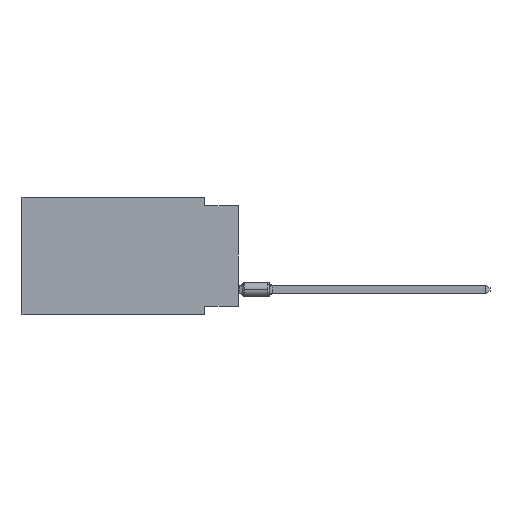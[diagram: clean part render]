
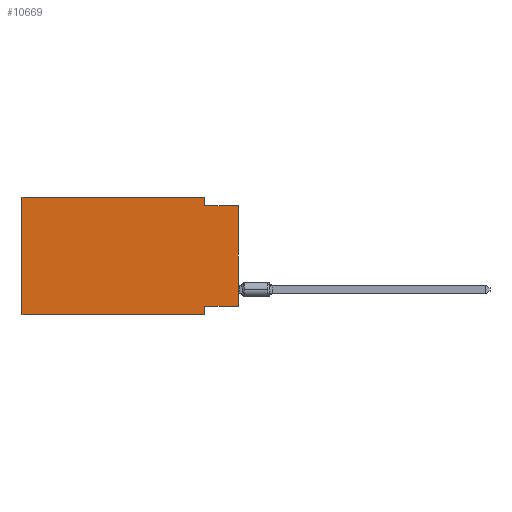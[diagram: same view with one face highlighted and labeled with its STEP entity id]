
A CAD part, left-side view. The second image highlights one B-rep face of the part: STEP entity #10669.
In plain terms, the highlighted planar face has unit normal (-1, 0, 0).
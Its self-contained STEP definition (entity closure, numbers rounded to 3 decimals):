
#193 = DIRECTION ( 'NONE',  ( 1., 0., 0. ) ) ;
#274 = CARTESIAN_POINT ( 'NONE',  ( 0., 16.383, -8.89 ) ) ;
#653 = CARTESIAN_POINT ( 'NONE',  ( 0., 2.54, -8.89 ) ) ;
#1124 = CARTESIAN_POINT ( 'NONE',  ( 0., 2.54, -8.255 ) ) ;
#1234 = EDGE_CURVE ( 'NONE', #23186, #7892, #2621, .T. ) ;
#1255 = DIRECTION ( 'NONE',  ( 0., 0., -1. ) ) ;
#1468 = VECTOR ( 'NONE', #2240, 1000. ) ;
#2240 = DIRECTION ( 'NONE',  ( 0., -1., 0. ) ) ;
#2472 = CARTESIAN_POINT ( 'NONE',  ( 0., 0., -8.255 ) ) ;
#2621 = LINE ( 'NONE', #274, #15415 ) ;
#3087 = VERTEX_POINT ( 'NONE', #1124 ) ;
#3174 = VECTOR ( 'NONE', #6211, 1000. ) ;
#4924 = ORIENTED_EDGE ( 'NONE', *, *, #26091, .F. ) ;
#5111 = EDGE_CURVE ( 'NONE', #9303, #13678, #6486, .T. ) ;
#5832 = AXIS2_PLACEMENT_3D ( 'NONE', #20250, #193, #18055 ) ;
#5965 = CARTESIAN_POINT ( 'NONE',  ( 0., 2.54, -0.635 ) ) ;
#6211 = DIRECTION ( 'NONE',  ( 0., 0., 1. ) ) ;
#6486 = LINE ( 'NONE', #13636, #1468 ) ;
#6857 = LINE ( 'NONE', #2472, #12995 ) ;
#7175 = CARTESIAN_POINT ( 'NONE',  ( 0., 2.54, 0. ) ) ;
#7892 = VERTEX_POINT ( 'NONE', #24386 ) ;
#8264 = LINE ( 'NONE', #26251, #3174 ) ;
#8518 = CARTESIAN_POINT ( 'NONE',  ( 0., 0., -0.635 ) ) ;
#8676 = VECTOR ( 'NONE', #22756, 1000. ) ;
#9214 = DIRECTION ( 'NONE',  ( 0., -1., 0. ) ) ;
#9303 = VERTEX_POINT ( 'NONE', #19679 ) ;
#9828 = DIRECTION ( 'NONE',  ( 0., 0., 1. ) ) ;
#10669 = ADVANCED_FACE ( 'NONE', ( #22589 ), #11321, .F. ) ;
#11321 = PLANE ( 'NONE',  #5832 ) ;
#11627 = VERTEX_POINT ( 'NONE', #5965 ) ;
#11881 = EDGE_CURVE ( 'NONE', #11627, #12589, #20565, .T. ) ;
#11915 = ORIENTED_EDGE ( 'NONE', *, *, #11881, .F. ) ;
#12589 = VERTEX_POINT ( 'NONE', #8518 ) ;
#12995 = VECTOR ( 'NONE', #17546, 1000. ) ;
#13097 = ORIENTED_EDGE ( 'NONE', *, *, #24279, .T. ) ;
#13636 = CARTESIAN_POINT ( 'NONE',  ( 0., 16.383, 0. ) ) ;
#13678 = VERTEX_POINT ( 'NONE', #28129 ) ;
#15415 = VECTOR ( 'NONE', #9214, 1000. ) ;
#15428 = EDGE_CURVE ( 'NONE', #23186, #9303, #27668, .T. ) ;
#16097 = DIRECTION ( 'NONE',  ( 0., 0., -1. ) ) ;
#16937 = EDGE_CURVE ( 'NONE', #3087, #7892, #27424, .T. ) ;
#17546 = DIRECTION ( 'NONE',  ( 0., 1., 0. ) ) ;
#18055 = DIRECTION ( 'NONE',  ( 0., 0., -1. ) ) ;
#18076 = CARTESIAN_POINT ( 'NONE',  ( 0., 0., -0.635 ) ) ;
#18197 = VECTOR ( 'NONE', #16097, 1000. ) ;
#19039 = CARTESIAN_POINT ( 'NONE',  ( 0., 16.383, 0. ) ) ;
#19333 = ORIENTED_EDGE ( 'NONE', *, *, #26439, .F. ) ;
#19371 = VECTOR ( 'NONE', #1255, 1000. ) ;
#19526 = VERTEX_POINT ( 'NONE', #24439 ) ;
#19636 = VECTOR ( 'NONE', #9828, 1000. ) ;
#19679 = CARTESIAN_POINT ( 'NONE',  ( 0., 16.383, 0. ) ) ;
#19741 = EDGE_LOOP ( 'NONE', ( #13097, #11915, #4924, #20662, #20695, #22804, #27108, #19333 ) ) ;
#20250 = CARTESIAN_POINT ( 'NONE',  ( 0., 16.383, 0. ) ) ;
#20565 = LINE ( 'NONE', #18076, #8676 ) ;
#20662 = ORIENTED_EDGE ( 'NONE', *, *, #5111, .F. ) ;
#20695 = ORIENTED_EDGE ( 'NONE', *, *, #15428, .F. ) ;
#20948 = LINE ( 'NONE', #7175, #18197 ) ;
#22589 = FACE_OUTER_BOUND ( 'NONE', #19741, .T. ) ;
#22756 = DIRECTION ( 'NONE',  ( 0., -1., 0. ) ) ;
#22804 = ORIENTED_EDGE ( 'NONE', *, *, #1234, .T. ) ;
#23186 = VERTEX_POINT ( 'NONE', #24157 ) ;
#24157 = CARTESIAN_POINT ( 'NONE',  ( 0., 16.383, -8.89 ) ) ;
#24279 = EDGE_CURVE ( 'NONE', #19526, #12589, #8264, .T. ) ;
#24386 = CARTESIAN_POINT ( 'NONE',  ( 0., 2.54, -8.89 ) ) ;
#24439 = CARTESIAN_POINT ( 'NONE',  ( 0., 0., -8.255 ) ) ;
#26091 = EDGE_CURVE ( 'NONE', #13678, #11627, #20948, .T. ) ;
#26251 = CARTESIAN_POINT ( 'NONE',  ( 0., 0., 0. ) ) ;
#26439 = EDGE_CURVE ( 'NONE', #19526, #3087, #6857, .T. ) ;
#27108 = ORIENTED_EDGE ( 'NONE', *, *, #16937, .F. ) ;
#27424 = LINE ( 'NONE', #653, #19371 ) ;
#27668 = LINE ( 'NONE', #19039, #19636 ) ;
#28129 = CARTESIAN_POINT ( 'NONE',  ( 0., 2.54, 0. ) ) ;
